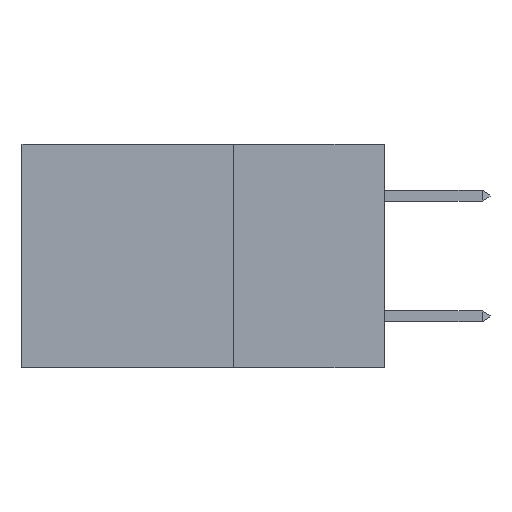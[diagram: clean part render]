
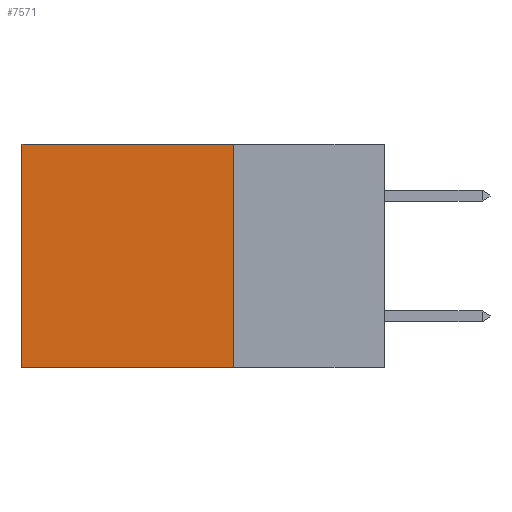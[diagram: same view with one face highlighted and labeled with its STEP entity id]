
A CAD part, left-side view. The second image highlights one B-rep face of the part: STEP entity #7571.
In plain terms, the highlighted planar face has unit normal (-1, 0, 0).
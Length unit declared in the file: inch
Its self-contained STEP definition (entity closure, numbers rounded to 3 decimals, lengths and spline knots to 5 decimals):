
#744 = ORIENTED_EDGE ( 'NONE', *, *, #16972, .T. ) ;
#1793 = CARTESIAN_POINT ( 'NONE',  ( 0.2875, 0.6, 0. ) ) ;
#2779 = VECTOR ( 'NONE', #8503, 39.37008 ) ;
#2782 = VECTOR ( 'NONE', #11103, 39.37008 ) ;
#2924 = CARTESIAN_POINT ( 'NONE',  ( 0.2875, 0.25, -0.37 ) ) ;
#3435 = CARTESIAN_POINT ( 'NONE',  ( 0.2875, 0.25, -0.37 ) ) ;
#4590 = ORIENTED_EDGE ( 'NONE', *, *, #12074, .F. ) ;
#5170 = CARTESIAN_POINT ( 'NONE',  ( 0.2875, 0.25, 0. ) ) ;
#5191 = DIRECTION ( 'NONE',  ( 1., 0., 0. ) ) ;
#5424 = AXIS2_PLACEMENT_3D ( 'NONE', #8046, #5191, #10671 ) ;
#7169 = LINE ( 'NONE', #2924, #2782 ) ;
#7429 = VECTOR ( 'NONE', #15406, 39.37008 ) ;
#7571 = ADVANCED_FACE ( 'NONE', ( #14426 ), #14769, .F. ) ;
#7943 = EDGE_CURVE ( 'NONE', #9415, #10917, #15790, .T. ) ;
#7968 = CARTESIAN_POINT ( 'NONE',  ( 0.2875, 0.6, -0.37 ) ) ;
#8046 = CARTESIAN_POINT ( 'NONE',  ( 0.2875, 0.25, 0. ) ) ;
#8503 = DIRECTION ( 'NONE',  ( 0., 0., -1. ) ) ;
#8758 = LINE ( 'NONE', #10080, #7429 ) ;
#8825 = VERTEX_POINT ( 'NONE', #7968 ) ;
#9415 = VERTEX_POINT ( 'NONE', #16508 ) ;
#9455 = EDGE_CURVE ( 'NONE', #12952, #8825, #7169, .T. ) ;
#9896 = CARTESIAN_POINT ( 'NONE',  ( 0.2875, 0.6, 0. ) ) ;
#10080 = CARTESIAN_POINT ( 'NONE',  ( 0.2875, 0.25, 0. ) ) ;
#10671 = DIRECTION ( 'NONE',  ( 0., 0., -1. ) ) ;
#10917 = VERTEX_POINT ( 'NONE', #1793 ) ;
#11103 = DIRECTION ( 'NONE',  ( 0., 1., 0. ) ) ;
#11854 = EDGE_LOOP ( 'NONE', ( #744, #14375, #4590, #14966 ) ) ;
#12074 = EDGE_CURVE ( 'NONE', #9415, #12952, #8758, .T. ) ;
#12952 = VERTEX_POINT ( 'NONE', #3435 ) ;
#12963 = VECTOR ( 'NONE', #14405, 39.37008 ) ;
#14375 = ORIENTED_EDGE ( 'NONE', *, *, #9455, .F. ) ;
#14405 = DIRECTION ( 'NONE',  ( 0., 1., 0. ) ) ;
#14426 = FACE_OUTER_BOUND ( 'NONE', #11854, .T. ) ;
#14769 = PLANE ( 'NONE',  #5424 ) ;
#14966 = ORIENTED_EDGE ( 'NONE', *, *, #7943, .T. ) ;
#15235 = LINE ( 'NONE', #9896, #2779 ) ;
#15406 = DIRECTION ( 'NONE',  ( 0., 0., -1. ) ) ;
#15790 = LINE ( 'NONE', #5170, #12963 ) ;
#16508 = CARTESIAN_POINT ( 'NONE',  ( 0.2875, 0.25, 0. ) ) ;
#16972 = EDGE_CURVE ( 'NONE', #10917, #8825, #15235, .T. ) ;
